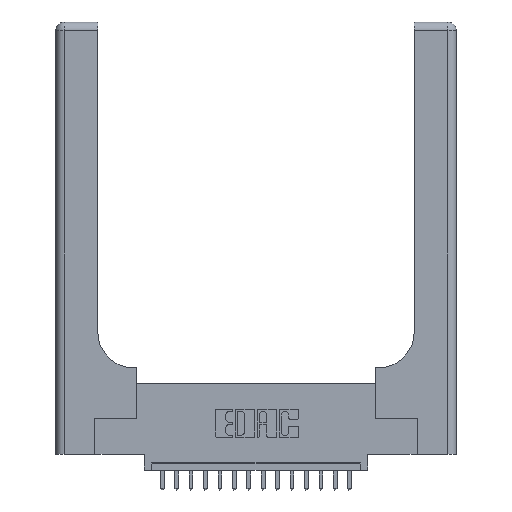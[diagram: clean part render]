
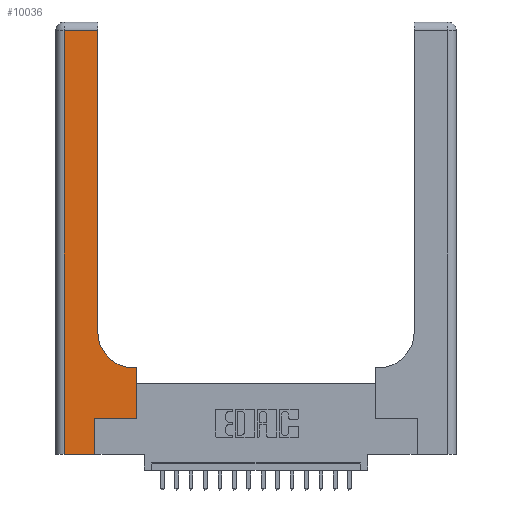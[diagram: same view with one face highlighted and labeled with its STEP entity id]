
A CAD part, top view. The second image highlights one B-rep face of the part: STEP entity #10036.
In plain terms, the highlighted planar face has unit normal (0, 0, 1).
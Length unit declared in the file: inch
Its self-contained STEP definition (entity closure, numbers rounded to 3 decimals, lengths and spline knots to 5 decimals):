
#163 = LINE ( 'NONE', #7904, #1559 ) ;
#1072 = CARTESIAN_POINT ( 'NONE',  ( 0.5585, 0.25, 0.37 ) ) ;
#1520 = CARTESIAN_POINT ( 'NONE',  ( 0.2915, 0.85, 0.37 ) ) ;
#1559 = VECTOR ( 'NONE', #14018, 39.37008 ) ;
#1602 = CARTESIAN_POINT ( 'NONE',  ( 0.5585, 0.25, 0.37 ) ) ;
#1655 = EDGE_LOOP ( 'NONE', ( #3024, #13865, #4513, #13136, #17661, #14565, #13840, #10325, #3733 ) ) ;
#1722 = LINE ( 'NONE', #1602, #13822 ) ;
#2038 = EDGE_CURVE ( 'NONE', #13060, #16388, #163, .T. ) ;
#2039 = DIRECTION ( 'NONE',  ( 0., 0., -1. ) ) ;
#2251 = CARTESIAN_POINT ( 'NONE',  ( 0., 2.94, 0.37 ) ) ;
#2280 = VECTOR ( 'NONE', #15480, 39.37008 ) ;
#2490 = CARTESIAN_POINT ( 'NONE',  ( 0.06, 0., 0.37 ) ) ;
#2705 = CARTESIAN_POINT ( 'NONE',  ( 0.5585, 0.6, 0.37 ) ) ;
#2822 = CARTESIAN_POINT ( 'NONE',  ( 0.06, 2.94, 0.37 ) ) ;
#3024 = ORIENTED_EDGE ( 'NONE', *, *, #12853, .T. ) ;
#3424 = CARTESIAN_POINT ( 'NONE',  ( 0.2915, 0.6, 0.37 ) ) ;
#3733 = ORIENTED_EDGE ( 'NONE', *, *, #12993, .T. ) ;
#4398 = DIRECTION ( 'NONE',  ( 1., 0., 0. ) ) ;
#4513 = ORIENTED_EDGE ( 'NONE', *, *, #7679, .T. ) ;
#4643 = EDGE_CURVE ( 'NONE', #8910, #11267, #17007, .T. ) ;
#5426 = VECTOR ( 'NONE', #19373, 39.37008 ) ;
#5592 = VECTOR ( 'NONE', #12539, 39.37008 ) ;
#5883 = CARTESIAN_POINT ( 'NONE',  ( 0., 0., 0.37 ) ) ;
#5910 = VECTOR ( 'NONE', #4398, 39.37008 ) ;
#6042 = CARTESIAN_POINT ( 'NONE',  ( 0.5415, 0.6, 0.37 ) ) ;
#6542 = CARTESIAN_POINT ( 'NONE',  ( 0., 3., 0.37 ) ) ;
#7443 = EDGE_CURVE ( 'NONE', #18342, #14415, #1722, .T. ) ;
#7679 = EDGE_CURVE ( 'NONE', #11267, #13867, #12850, .T. ) ;
#7824 = DIRECTION ( 'NONE',  ( 0., 1., 0. ) ) ;
#7904 = CARTESIAN_POINT ( 'NONE',  ( 0.269, 0., 0.37 ) ) ;
#8765 = CARTESIAN_POINT ( 'NONE',  ( 0.269, 0., 0.37 ) ) ;
#8910 = VERTEX_POINT ( 'NONE', #15625 ) ;
#9070 = VECTOR ( 'NONE', #10230, 39.37008 ) ;
#9293 = DIRECTION ( 'NONE',  ( 0., -1., 0. ) ) ;
#10036 = ADVANCED_FACE ( 'NONE', ( #13285 ), #14279, .F. ) ;
#10230 = DIRECTION ( 'NONE',  ( 1., 0., 0. ) ) ;
#10325 = ORIENTED_EDGE ( 'NONE', *, *, #12286, .T. ) ;
#10423 = EDGE_CURVE ( 'NONE', #16388, #18342, #17295, .T. ) ;
#10506 = LINE ( 'NONE', #12348, #5592 ) ;
#10608 = CARTESIAN_POINT ( 'NONE',  ( 0.06, 3., 0.37 ) ) ;
#10719 = LINE ( 'NONE', #5883, #9070 ) ;
#11267 = VERTEX_POINT ( 'NONE', #2822 ) ;
#12233 = LINE ( 'NONE', #3424, #2280 ) ;
#12286 = EDGE_CURVE ( 'NONE', #14415, #15619, #12233, .T. ) ;
#12348 = CARTESIAN_POINT ( 'NONE',  ( 0.2915, 3., 0.37 ) ) ;
#12539 = DIRECTION ( 'NONE',  ( 0., 1., 0. ) ) ;
#12850 = LINE ( 'NONE', #10608, #17863 ) ;
#12853 = EDGE_CURVE ( 'NONE', #17938, #8910, #10506, .T. ) ;
#12993 = EDGE_CURVE ( 'NONE', #15619, #17938, #13633, .T. ) ;
#13060 = VERTEX_POINT ( 'NONE', #8765 ) ;
#13136 = ORIENTED_EDGE ( 'NONE', *, *, #13523, .T. ) ;
#13285 = FACE_OUTER_BOUND ( 'NONE', #1655, .T. ) ;
#13523 = EDGE_CURVE ( 'NONE', #13867, #13060, #10719, .T. ) ;
#13633 = CIRCLE ( 'NONE', #15080, 0.25 ) ;
#13822 = VECTOR ( 'NONE', #7824, 39.37008 ) ;
#13840 = ORIENTED_EDGE ( 'NONE', *, *, #7443, .T. ) ;
#13865 = ORIENTED_EDGE ( 'NONE', *, *, #4643, .T. ) ;
#13867 = VERTEX_POINT ( 'NONE', #2490 ) ;
#14018 = DIRECTION ( 'NONE',  ( 0., 1., 0. ) ) ;
#14279 = PLANE ( 'NONE',  #17767 ) ;
#14349 = DIRECTION ( 'NONE',  ( -1., 0., 0. ) ) ;
#14415 = VERTEX_POINT ( 'NONE', #2705 ) ;
#14565 = ORIENTED_EDGE ( 'NONE', *, *, #10423, .T. ) ;
#14612 = CARTESIAN_POINT ( 'NONE',  ( 0.5415, 0.85, 0.37 ) ) ;
#15080 = AXIS2_PLACEMENT_3D ( 'NONE', #14612, #2039, #17770 ) ;
#15480 = DIRECTION ( 'NONE',  ( -1., 0., 0. ) ) ;
#15619 = VERTEX_POINT ( 'NONE', #6042 ) ;
#15625 = CARTESIAN_POINT ( 'NONE',  ( 0.2915, 2.94, 0.37 ) ) ;
#15825 = DIRECTION ( 'NONE',  ( 0., 0., -1. ) ) ;
#16388 = VERTEX_POINT ( 'NONE', #16935 ) ;
#16935 = CARTESIAN_POINT ( 'NONE',  ( 0.269, 0.25, 0.37 ) ) ;
#17007 = LINE ( 'NONE', #2251, #5426 ) ;
#17295 = LINE ( 'NONE', #17986, #5910 ) ;
#17661 = ORIENTED_EDGE ( 'NONE', *, *, #2038, .T. ) ;
#17767 = AXIS2_PLACEMENT_3D ( 'NONE', #6542, #15825, #14349 ) ;
#17770 = DIRECTION ( 'NONE',  ( 1., 0., 0. ) ) ;
#17863 = VECTOR ( 'NONE', #9293, 39.37008 ) ;
#17938 = VERTEX_POINT ( 'NONE', #1520 ) ;
#17986 = CARTESIAN_POINT ( 'NONE',  ( 0.269, 0.25, 0.37 ) ) ;
#18342 = VERTEX_POINT ( 'NONE', #1072 ) ;
#19373 = DIRECTION ( 'NONE',  ( -1., 0., 0. ) ) ;
